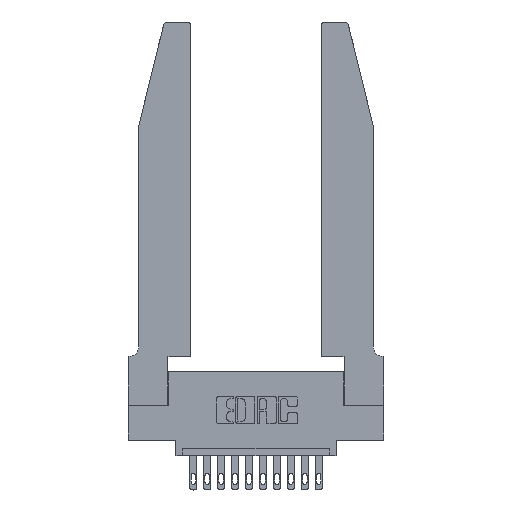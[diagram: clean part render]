
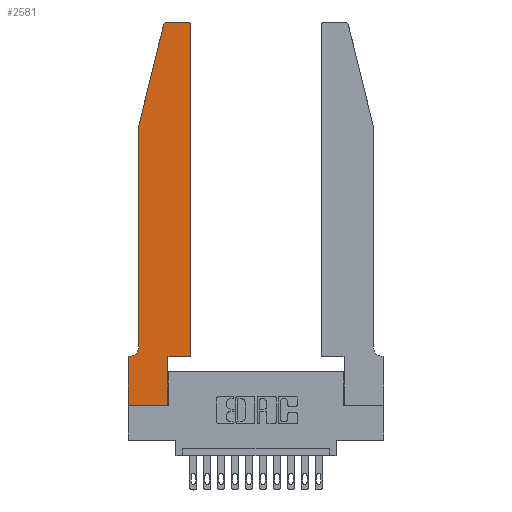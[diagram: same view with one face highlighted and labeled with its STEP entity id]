
A CAD part, top view. The second image highlights one B-rep face of the part: STEP entity #2581.
In plain terms, the highlighted planar face has unit normal (0, 0, 1).
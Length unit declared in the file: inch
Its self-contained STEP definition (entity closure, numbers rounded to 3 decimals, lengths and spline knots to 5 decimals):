
#454 = ORIENTED_EDGE ( 'NONE', *, *, #10784, .T. ) ;
#817 = LINE ( 'NONE', #15081, #16286 ) ;
#1091 = CARTESIAN_POINT ( 'NONE',  ( 0.4505, 0.35, 0.37 ) ) ;
#1211 = VERTEX_POINT ( 'NONE', #5028 ) ;
#1320 = AXIS2_PLACEMENT_3D ( 'NONE', #11980, #10696, #10809 ) ;
#1887 = LINE ( 'NONE', #2862, #12320 ) ;
#1946 = VERTEX_POINT ( 'NONE', #3735 ) ;
#2211 = CARTESIAN_POINT ( 'NONE',  ( 0.2865, 0.35, 0.37 ) ) ;
#2251 = ORIENTED_EDGE ( 'NONE', *, *, #8678, .T. ) ;
#2261 = LINE ( 'NONE', #14131, #5825 ) ;
#2399 = VERTEX_POINT ( 'NONE', #13893 ) ;
#2430 = EDGE_CURVE ( 'NONE', #14334, #5652, #9666, .T. ) ;
#2484 = VECTOR ( 'NONE', #5389, 39.37008 ) ;
#2565 = CARTESIAN_POINT ( 'NONE',  ( 0.0755, 0.35, 0.37 ) ) ;
#2581 = ADVANCED_FACE ( 'NONE', ( #15922 ), #9387, .T. ) ;
#2754 = LINE ( 'NONE', #13412, #10779 ) ;
#2862 = CARTESIAN_POINT ( 'NONE',  ( 0.4505, 0.35, 0.37 ) ) ;
#2931 = ORIENTED_EDGE ( 'NONE', *, *, #16199, .T. ) ;
#3099 = EDGE_CURVE ( 'NONE', #1946, #14334, #15314, .T. ) ;
#3157 = VECTOR ( 'NONE', #5599, 39.37008 ) ;
#3419 = VERTEX_POINT ( 'NONE', #6066 ) ;
#3436 = ORIENTED_EDGE ( 'NONE', *, *, #2430, .T. ) ;
#3735 = CARTESIAN_POINT ( 'NONE',  ( 0.0755, 0.42, 0.37 ) ) ;
#3841 = VERTEX_POINT ( 'NONE', #7802 ) ;
#3951 = LINE ( 'NONE', #13302, #3157 ) ;
#4373 = DIRECTION ( 'NONE',  ( -1., 0., 0. ) ) ;
#4413 = VECTOR ( 'NONE', #16473, 39.37008 ) ;
#4544 = VERTEX_POINT ( 'NONE', #11747 ) ;
#5028 = CARTESIAN_POINT ( 'NONE',  ( 0.4505, 2.72, 0.37 ) ) ;
#5359 = VERTEX_POINT ( 'NONE', #10821 ) ;
#5389 = DIRECTION ( 'NONE',  ( -1., 0., 0. ) ) ;
#5391 = ORIENTED_EDGE ( 'NONE', *, *, #10571, .T. ) ;
#5599 = DIRECTION ( 'NONE',  ( 0., -1., 0. ) ) ;
#5652 = VERTEX_POINT ( 'NONE', #14898 ) ;
#5825 = VECTOR ( 'NONE', #6408, 39.37008 ) ;
#5920 = EDGE_CURVE ( 'NONE', #2399, #1211, #1887, .T. ) ;
#6066 = CARTESIAN_POINT ( 'NONE',  ( 0.2865, 0., 0.37 ) ) ;
#6408 = DIRECTION ( 'NONE',  ( 0., 1., 0. ) ) ;
#6409 = CIRCLE ( 'NONE', #1320, 0.03 ) ;
#6620 = VECTOR ( 'NONE', #16296, 39.37008 ) ;
#7230 = AXIS2_PLACEMENT_3D ( 'NONE', #10595, #12054, #4373 ) ;
#7281 = CARTESIAN_POINT ( 'NONE',  ( 0.0055, 0.35, 0.37 ) ) ;
#7283 = CARTESIAN_POINT ( 'NONE',  ( 0., 0., 0.37 ) ) ;
#7412 = ORIENTED_EDGE ( 'NONE', *, *, #15642, .T. ) ;
#7527 = EDGE_CURVE ( 'NONE', #5359, #3841, #817, .T. ) ;
#7802 = CARTESIAN_POINT ( 'NONE',  ( 0.0755, 2., 0.37 ) ) ;
#8276 = ORIENTED_EDGE ( 'NONE', *, *, #15939, .T. ) ;
#8491 = DIRECTION ( 'NONE',  ( -0.239, -0.971, 0. ) ) ;
#8678 = EDGE_CURVE ( 'NONE', #1211, #9190, #16052, .T. ) ;
#8702 = ORIENTED_EDGE ( 'NONE', *, *, #5920, .T. ) ;
#8728 = AXIS2_PLACEMENT_3D ( 'NONE', #13478, #14774, #10674 ) ;
#9190 = VERTEX_POINT ( 'NONE', #10228 ) ;
#9209 = DIRECTION ( 'NONE',  ( 0., 0., 1. ) ) ;
#9387 = PLANE ( 'NONE',  #8728 ) ;
#9666 = LINE ( 'NONE', #2565, #2484 ) ;
#9793 = ORIENTED_EDGE ( 'NONE', *, *, #7527, .T. ) ;
#10165 = CARTESIAN_POINT ( 'NONE',  ( 0.284, 2.75, 0.37 ) ) ;
#10228 = CARTESIAN_POINT ( 'NONE',  ( 0.4205, 2.75, 0.37 ) ) ;
#10571 = EDGE_CURVE ( 'NONE', #13698, #5359, #6409, .T. ) ;
#10595 = CARTESIAN_POINT ( 'NONE',  ( 0.0055, 0.42, 0.37 ) ) ;
#10674 = DIRECTION ( 'NONE',  ( 1., 0., 0. ) ) ;
#10685 = CARTESIAN_POINT ( 'NONE',  ( 0., 0., 0.37 ) ) ;
#10696 = DIRECTION ( 'NONE',  ( 0., 0., 1. ) ) ;
#10779 = VECTOR ( 'NONE', #14602, 39.37008 ) ;
#10784 = EDGE_CURVE ( 'NONE', #12948, #2399, #14656, .T. ) ;
#10809 = DIRECTION ( 'NONE',  ( 1., 0., 0. ) ) ;
#10821 = CARTESIAN_POINT ( 'NONE',  ( 0.25487, 2.72718, 0.37 ) ) ;
#10851 = DIRECTION ( 'NONE',  ( 1., 0., 0. ) ) ;
#10954 = DIRECTION ( 'NONE',  ( 0., 1., 0. ) ) ;
#11214 = ORIENTED_EDGE ( 'NONE', *, *, #3099, .T. ) ;
#11747 = CARTESIAN_POINT ( 'NONE',  ( 0., 0., 0.37 ) ) ;
#11970 = EDGE_LOOP ( 'NONE', ( #12265, #5391, #9793, #12837, #11214, #3436, #2931, #8276, #7412, #454, #8702, #2251 ) ) ;
#11980 = CARTESIAN_POINT ( 'NONE',  ( 0.284, 2.72, 0.37 ) ) ;
#12054 = DIRECTION ( 'NONE',  ( 0., 0., -1. ) ) ;
#12265 = ORIENTED_EDGE ( 'NONE', *, *, #12764, .T. ) ;
#12320 = VECTOR ( 'NONE', #10954, 39.37008 ) ;
#12747 = EDGE_CURVE ( 'NONE', #3841, #1946, #3951, .T. ) ;
#12764 = EDGE_CURVE ( 'NONE', #9190, #13698, #2754, .T. ) ;
#12837 = ORIENTED_EDGE ( 'NONE', *, *, #12747, .T. ) ;
#12948 = VERTEX_POINT ( 'NONE', #2211 ) ;
#13302 = CARTESIAN_POINT ( 'NONE',  ( 0.0755, 2., 0.37 ) ) ;
#13412 = CARTESIAN_POINT ( 'NONE',  ( 0.2605, 2.75, 0.37 ) ) ;
#13478 = CARTESIAN_POINT ( 'NONE',  ( 0., 0.35, 0.37 ) ) ;
#13698 = VERTEX_POINT ( 'NONE', #10165 ) ;
#13893 = CARTESIAN_POINT ( 'NONE',  ( 0.4505, 0.35, 0.37 ) ) ;
#14131 = CARTESIAN_POINT ( 'NONE',  ( 0.2865, 0.35, 0.37 ) ) ;
#14334 = VERTEX_POINT ( 'NONE', #7281 ) ;
#14415 = DIRECTION ( 'NONE',  ( 1., 0., 0. ) ) ;
#14602 = DIRECTION ( 'NONE',  ( -1., 0., 0. ) ) ;
#14656 = LINE ( 'NONE', #1091, #4413 ) ;
#14672 = LINE ( 'NONE', #10685, #16291 ) ;
#14774 = DIRECTION ( 'NONE',  ( 0., 0., 1. ) ) ;
#14898 = CARTESIAN_POINT ( 'NONE',  ( 0., 0.35, 0.37 ) ) ;
#14955 = AXIS2_PLACEMENT_3D ( 'NONE', #15647, #9209, #14415 ) ;
#15081 = CARTESIAN_POINT ( 'NONE',  ( 0.0755, 2., 0.37 ) ) ;
#15289 = LINE ( 'NONE', #7283, #6620 ) ;
#15314 = CIRCLE ( 'NONE', #7230, 0.07 ) ;
#15642 = EDGE_CURVE ( 'NONE', #3419, #12948, #2261, .T. ) ;
#15647 = CARTESIAN_POINT ( 'NONE',  ( 0.4205, 2.72, 0.37 ) ) ;
#15922 = FACE_OUTER_BOUND ( 'NONE', #11970, .T. ) ;
#15939 = EDGE_CURVE ( 'NONE', #4544, #3419, #14672, .T. ) ;
#16052 = CIRCLE ( 'NONE', #14955, 0.03 ) ;
#16199 = EDGE_CURVE ( 'NONE', #5652, #4544, #15289, .T. ) ;
#16286 = VECTOR ( 'NONE', #8491, 39.37008 ) ;
#16291 = VECTOR ( 'NONE', #10851, 39.37008 ) ;
#16296 = DIRECTION ( 'NONE',  ( 0., -1., 0. ) ) ;
#16473 = DIRECTION ( 'NONE',  ( 1., 0., 0. ) ) ;
